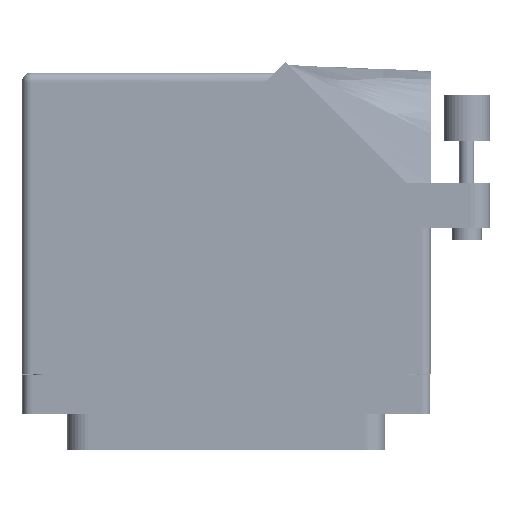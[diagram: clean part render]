
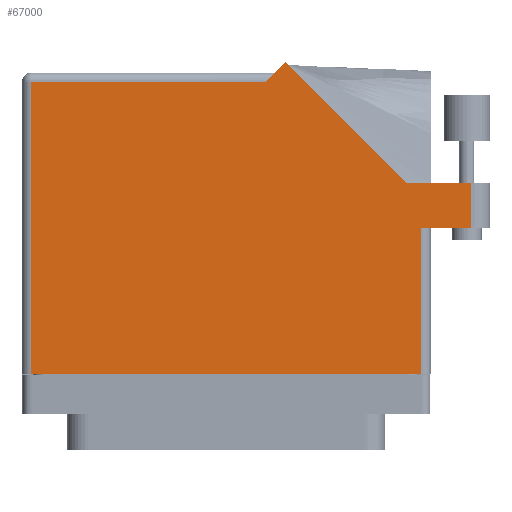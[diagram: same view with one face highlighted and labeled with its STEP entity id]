
A CAD part, front view. The second image highlights one B-rep face of the part: STEP entity #67000.
In plain terms, the highlighted face is planar.
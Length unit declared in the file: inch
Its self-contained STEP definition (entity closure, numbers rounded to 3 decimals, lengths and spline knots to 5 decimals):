
#198 = EDGE_LOOP ( 'NONE', ( #76887, #51854, #15442, #59985, #59390, #18398, #55062, #23877, #4110 ) ) ;
#1755 = EDGE_CURVE ( 'NONE', #15379, #12144, #56278, .T. ) ;
#2356 = CARTESIAN_POINT ( 'NONE',  ( 1.6525, 1.187, 0.765 ) ) ;
#2737 = EDGE_CURVE ( 'NONE', #46446, #15379, #28861, .T. ) ;
#3919 = CARTESIAN_POINT ( 'NONE',  ( 0.2655, 1.868, 0.765 ) ) ;
#4110 = ORIENTED_EDGE ( 'NONE', *, *, #2737, .T. ) ;
#6356 = CARTESIAN_POINT ( 'NONE',  ( -1.3155, 1.868, 0.765 ) ) ;
#6630 = VERTEX_POINT ( 'NONE', #48681 ) ;
#6672 = VERTEX_POINT ( 'NONE', #85088 ) ;
#7319 = VECTOR ( 'NONE', #40894, 39.37008 ) ;
#12144 = VERTEX_POINT ( 'NONE', #53246 ) ;
#14898 = CARTESIAN_POINT ( 'NONE',  ( 1.3155, 0.88, 0.765 ) ) ;
#15085 = EDGE_CURVE ( 'NONE', #6630, #46446, #26341, .T. ) ;
#15379 = VERTEX_POINT ( 'NONE', #14898 ) ;
#15442 = ORIENTED_EDGE ( 'NONE', *, *, #43844, .T. ) ;
#15598 = EDGE_CURVE ( 'NONE', #6672, #50297, #36230, .T. ) ;
#16535 = VERTEX_POINT ( 'NONE', #2356 ) ;
#17787 = CARTESIAN_POINT ( 'NONE',  ( 1.21192, 1.187, 0.765 ) ) ;
#18295 = CARTESIAN_POINT ( 'NONE',  ( 0.3275, 1.93, 0.765 ) ) ;
#18398 = ORIENTED_EDGE ( 'NONE', *, *, #84183, .T. ) ;
#18431 = DIRECTION ( 'NONE',  ( -1., 0., 0. ) ) ;
#19077 = LINE ( 'NONE', #71546, #58318 ) ;
#21431 = FACE_OUTER_BOUND ( 'NONE', #198, .T. ) ;
#22006 = CARTESIAN_POINT ( 'NONE',  ( 1.6525, 1.187, 0.765 ) ) ;
#23877 = ORIENTED_EDGE ( 'NONE', *, *, #15085, .T. ) ;
#24008 = DIRECTION ( 'NONE',  ( -1., 0., 0. ) ) ;
#24868 = CARTESIAN_POINT ( 'NONE',  ( 1.3775, 0.88, 0.765 ) ) ;
#26341 = LINE ( 'NONE', #48036, #7319 ) ;
#27035 = DIRECTION ( 'NONE',  ( 1., 0., 0. ) ) ;
#28861 = LINE ( 'NONE', #40994, #65709 ) ;
#29939 = LINE ( 'NONE', #22006, #62413 ) ;
#34635 = VECTOR ( 'NONE', #24008, 39.37008 ) ;
#36230 = LINE ( 'NONE', #18295, #69653 ) ;
#36578 = EDGE_CURVE ( 'NONE', #70726, #6672, #61397, .T. ) ;
#40544 = VECTOR ( 'NONE', #27035, 39.37008 ) ;
#40894 = DIRECTION ( 'NONE',  ( 1., 0., 0. ) ) ;
#40994 = CARTESIAN_POINT ( 'NONE',  ( 1.3155, 0.88, 0.765 ) ) ;
#43844 = EDGE_CURVE ( 'NONE', #16535, #70726, #75977, .T. ) ;
#46446 = VERTEX_POINT ( 'NONE', #51231 ) ;
#48036 = CARTESIAN_POINT ( 'NONE',  ( -1.3775, -0.1, 0.765 ) ) ;
#48681 = CARTESIAN_POINT ( 'NONE',  ( -1.3155, -0.1, 0.765 ) ) ;
#50297 = VERTEX_POINT ( 'NONE', #3919 ) ;
#51231 = CARTESIAN_POINT ( 'NONE',  ( 1.3155, -0.1, 0.765 ) ) ;
#51854 = ORIENTED_EDGE ( 'NONE', *, *, #81334, .T. ) ;
#53246 = CARTESIAN_POINT ( 'NONE',  ( 1.6525, 0.88, 0.765 ) ) ;
#53270 = CARTESIAN_POINT ( 'NONE',  ( 1.7775, 1.187, 0.765 ) ) ;
#53478 = DIRECTION ( 'NONE',  ( 0., 0., -1. ) ) ;
#55062 = ORIENTED_EDGE ( 'NONE', *, *, #67454, .T. ) ;
#56278 = LINE ( 'NONE', #24868, #40544 ) ;
#57023 = AXIS2_PLACEMENT_3D ( 'NONE', #90205, #53478, #18431 ) ;
#58318 = VECTOR ( 'NONE', #86611, 39.37008 ) ;
#59390 = ORIENTED_EDGE ( 'NONE', *, *, #15598, .T. ) ;
#59985 = ORIENTED_EDGE ( 'NONE', *, *, #36578, .T. ) ;
#61397 = LINE ( 'NONE', #70104, #77269 ) ;
#61487 = LINE ( 'NONE', #87987, #34635 ) ;
#62413 = VECTOR ( 'NONE', #88420, 39.37008 ) ;
#65709 = VECTOR ( 'NONE', #80500, 39.37008 ) ;
#67000 = ADVANCED_FACE ( 'NONE', ( #21431 ), #76424, .F. ) ;
#67454 = EDGE_CURVE ( 'NONE', #89883, #6630, #19077, .T. ) ;
#69653 = VECTOR ( 'NONE', #75945, 39.37008 ) ;
#70104 = CARTESIAN_POINT ( 'NONE',  ( 1.21192, 1.187, 0.765 ) ) ;
#70726 = VERTEX_POINT ( 'NONE', #17787 ) ;
#71546 = CARTESIAN_POINT ( 'NONE',  ( -1.3155, -0.1, 0.765 ) ) ;
#75945 = DIRECTION ( 'NONE',  ( -0.707, -0.707, 0. ) ) ;
#75977 = LINE ( 'NONE', #53270, #90559 ) ;
#76424 = PLANE ( 'NONE',  #57023 ) ;
#76887 = ORIENTED_EDGE ( 'NONE', *, *, #1755, .T. ) ;
#77269 = VECTOR ( 'NONE', #91747, 39.37008 ) ;
#80500 = DIRECTION ( 'NONE',  ( 0., 1., 0. ) ) ;
#81334 = EDGE_CURVE ( 'NONE', #12144, #16535, #29939, .T. ) ;
#83118 = DIRECTION ( 'NONE',  ( -1., 0., 0. ) ) ;
#84183 = EDGE_CURVE ( 'NONE', #50297, #89883, #61487, .T. ) ;
#85088 = CARTESIAN_POINT ( 'NONE',  ( 0.39821, 2.00071, 0.765 ) ) ;
#86611 = DIRECTION ( 'NONE',  ( 0., -1., 0. ) ) ;
#87987 = CARTESIAN_POINT ( 'NONE',  ( -1.3775, 1.868, 0.765 ) ) ;
#88420 = DIRECTION ( 'NONE',  ( 0., 1., 0. ) ) ;
#89883 = VERTEX_POINT ( 'NONE', #6356 ) ;
#90205 = CARTESIAN_POINT ( 'NONE',  ( -1.3775, 1.93, 0.765 ) ) ;
#90559 = VECTOR ( 'NONE', #83118, 39.37008 ) ;
#91747 = DIRECTION ( 'NONE',  ( -0.707, 0.707, 0. ) ) ;
